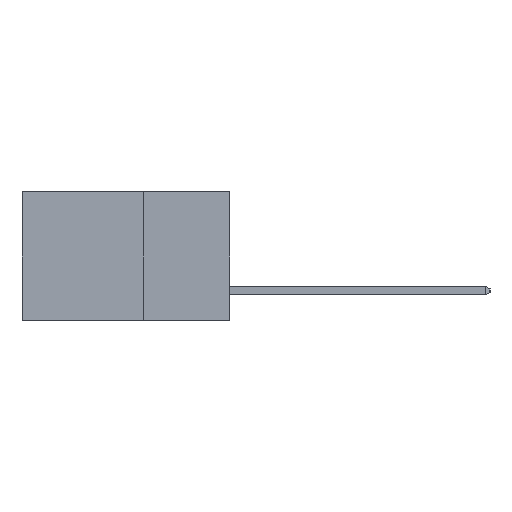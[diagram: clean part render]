
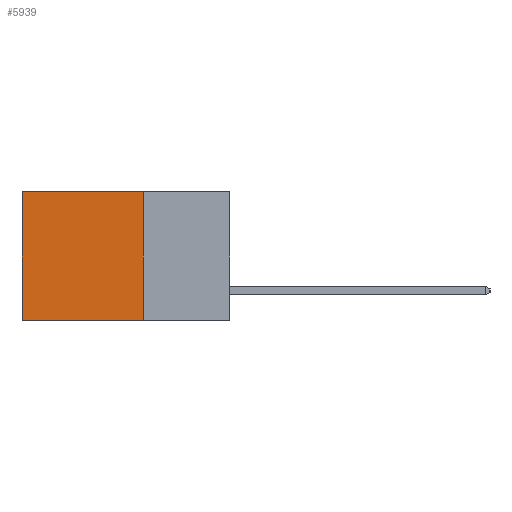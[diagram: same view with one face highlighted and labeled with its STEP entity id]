
A CAD part, left-side view. The second image highlights one B-rep face of the part: STEP entity #5939.
In plain terms, the highlighted planar face has unit normal (-1, 0, 0).
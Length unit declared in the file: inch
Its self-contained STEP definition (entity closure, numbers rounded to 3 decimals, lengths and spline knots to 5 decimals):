
#540 = EDGE_CURVE ( 'NONE', #10096, #10653, #12601, .T. ) ;
#948 = VERTEX_POINT ( 'NONE', #8910 ) ;
#1335 = LINE ( 'NONE', #4811, #7999 ) ;
#2377 = EDGE_LOOP ( 'NONE', ( #11157, #11917, #4059, #11848 ) ) ;
#2453 = CARTESIAN_POINT ( 'NONE',  ( 0.2615, 0.6, -0.37 ) ) ;
#2765 = CARTESIAN_POINT ( 'NONE',  ( 0.2615, 0.25, -0.37 ) ) ;
#3369 = CARTESIAN_POINT ( 'NONE',  ( 0.2615, 0.25, -0.37 ) ) ;
#3839 = DIRECTION ( 'NONE',  ( 0., 0., -1. ) ) ;
#4059 = ORIENTED_EDGE ( 'NONE', *, *, #13325, .F. ) ;
#4811 = CARTESIAN_POINT ( 'NONE',  ( 0.2615, 0.25, 0. ) ) ;
#5453 = VECTOR ( 'NONE', #11993, 39.37008 ) ;
#5939 = ADVANCED_FACE ( 'NONE', ( #6799 ), #13387, .F. ) ;
#6537 = CARTESIAN_POINT ( 'NONE',  ( 0.2615, 0.6, -0.37 ) ) ;
#6799 = FACE_OUTER_BOUND ( 'NONE', #2377, .T. ) ;
#7922 = CARTESIAN_POINT ( 'NONE',  ( 0.2615, 0.25, -0.37 ) ) ;
#7999 = VECTOR ( 'NONE', #15186, 39.37008 ) ;
#8154 = EDGE_CURVE ( 'NONE', #16739, #10653, #13716, .T. ) ;
#8430 = AXIS2_PLACEMENT_3D ( 'NONE', #12706, #12652, #12564 ) ;
#8910 = CARTESIAN_POINT ( 'NONE',  ( 0.2615, 0.25, 0. ) ) ;
#9505 = VECTOR ( 'NONE', #10674, 39.37008 ) ;
#9709 = LINE ( 'NONE', #2765, #5453 ) ;
#10096 = VERTEX_POINT ( 'NONE', #7922 ) ;
#10244 = VECTOR ( 'NONE', #3839, 39.37008 ) ;
#10653 = VERTEX_POINT ( 'NONE', #6537 ) ;
#10674 = DIRECTION ( 'NONE',  ( 0., 1., 0. ) ) ;
#11157 = ORIENTED_EDGE ( 'NONE', *, *, #8154, .T. ) ;
#11848 = ORIENTED_EDGE ( 'NONE', *, *, #12962, .T. ) ;
#11917 = ORIENTED_EDGE ( 'NONE', *, *, #540, .F. ) ;
#11993 = DIRECTION ( 'NONE',  ( 0., 0., -1. ) ) ;
#12564 = DIRECTION ( 'NONE',  ( 0., 0., -1. ) ) ;
#12601 = LINE ( 'NONE', #3369, #9505 ) ;
#12652 = DIRECTION ( 'NONE',  ( 1., 0., 0. ) ) ;
#12706 = CARTESIAN_POINT ( 'NONE',  ( 0.2615, 0.25, -0.37 ) ) ;
#12962 = EDGE_CURVE ( 'NONE', #948, #16739, #1335, .T. ) ;
#13325 = EDGE_CURVE ( 'NONE', #948, #10096, #9709, .T. ) ;
#13387 = PLANE ( 'NONE',  #8430 ) ;
#13716 = LINE ( 'NONE', #2453, #10244 ) ;
#15186 = DIRECTION ( 'NONE',  ( 0., 1., 0. ) ) ;
#15572 = CARTESIAN_POINT ( 'NONE',  ( 0.2615, 0.6, 0. ) ) ;
#16739 = VERTEX_POINT ( 'NONE', #15572 ) ;
